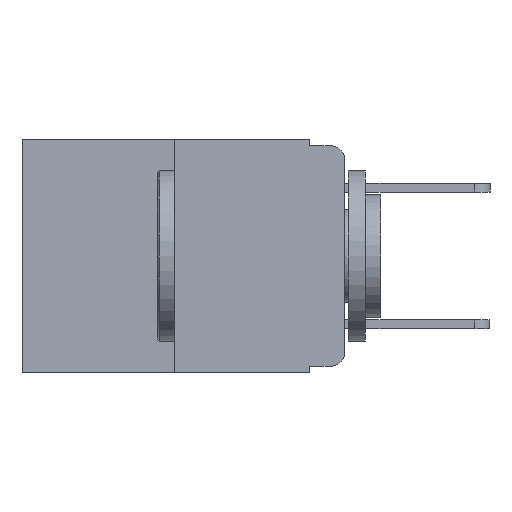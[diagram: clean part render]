
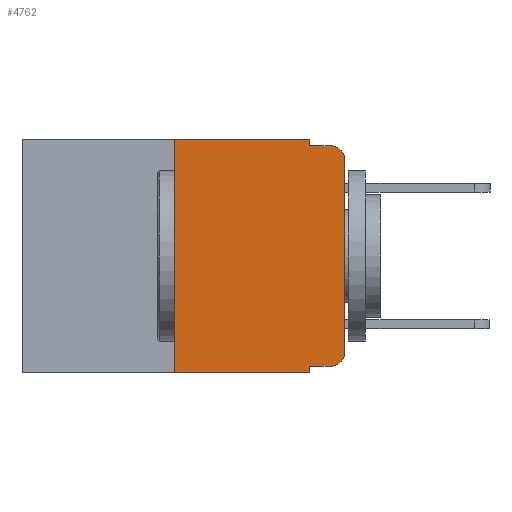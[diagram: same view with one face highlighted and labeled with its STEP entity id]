
A CAD part, left-side view. The second image highlights one B-rep face of the part: STEP entity #4762.
In plain terms, the highlighted planar face has unit normal (-1, 0, 0).
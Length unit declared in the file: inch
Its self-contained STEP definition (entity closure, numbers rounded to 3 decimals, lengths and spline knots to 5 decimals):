
#16 = ORIENTED_EDGE ( 'NONE', *, *, #5160, .F. ) ;
#153 = ORIENTED_EDGE ( 'NONE', *, *, #15971, .F. ) ;
#189 = AXIS2_PLACEMENT_3D ( 'NONE', #8895, #695, #12003 ) ;
#203 = ORIENTED_EDGE ( 'NONE', *, *, #5187, .F. ) ;
#223 = ORIENTED_EDGE ( 'NONE', *, *, #11264, .T. ) ;
#386 = VECTOR ( 'NONE', #772, 39.37008 ) ;
#425 = CIRCLE ( 'NONE', #189, 0.02 ) ;
#486 = ORIENTED_EDGE ( 'NONE', *, *, #5216, .F. ) ;
#529 = ORIENTED_EDGE ( 'NONE', *, *, #5248, .T. ) ;
#695 = DIRECTION ( 'NONE',  ( -1., 0., 0. ) ) ;
#772 = DIRECTION ( 'NONE',  ( 0., 0., 1. ) ) ;
#849 = CARTESIAN_POINT ( 'NONE',  ( 0., 0.051, -0.343 ) ) ;
#901 = ORIENTED_EDGE ( 'NONE', *, *, #5281, .T. ) ;
#1326 = VERTEX_POINT ( 'NONE', #10271 ) ;
#1379 = CARTESIAN_POINT ( 'NONE',  ( 0., 0.02, -0.333 ) ) ;
#1404 = CARTESIAN_POINT ( 'NONE',  ( 0., 0.051, -0.01 ) ) ;
#1521 = ORIENTED_EDGE ( 'NONE', *, *, #3767, .T. ) ;
#2048 = VECTOR ( 'NONE', #12965, 39.37008 ) ;
#2095 = DIRECTION ( 'NONE',  ( 1., 0., 0. ) ) ;
#2375 = EDGE_LOOP ( 'NONE', ( #1521, #2548, #7678, #16, #153, #203, #223, #486, #529, #901 ) ) ;
#2379 = VERTEX_POINT ( 'NONE', #1379 ) ;
#2535 = CARTESIAN_POINT ( 'NONE',  ( 0., 0.051, -0.01 ) ) ;
#2548 = ORIENTED_EDGE ( 'NONE', *, *, #4311, .T. ) ;
#2632 = VERTEX_POINT ( 'NONE', #16385 ) ;
#3217 = VECTOR ( 'NONE', #9694, 39.37008 ) ;
#3767 = EDGE_CURVE ( 'NONE', #12517, #16315, #13210, .T. ) ;
#3770 = AXIS2_PLACEMENT_3D ( 'NONE', #10000, #2095, #11197 ) ;
#3823 = FACE_OUTER_BOUND ( 'NONE', #2375, .T. ) ;
#4311 = EDGE_CURVE ( 'NONE', #16315, #15438, #425, .T. ) ;
#4473 = CARTESIAN_POINT ( 'NONE',  ( 0., 0.02, -0.01 ) ) ;
#4698 = VERTEX_POINT ( 'NONE', #849 ) ;
#4762 = ADVANCED_FACE ( 'NONE', ( #3823 ), #6247, .F. ) ;
#4824 = EDGE_CURVE ( 'NONE', #13267, #15438, #15745, .T. ) ;
#5026 = DIRECTION ( 'NONE',  ( 0., 0., -1. ) ) ;
#5160 = EDGE_CURVE ( 'NONE', #1326, #13267, #11373, .T. ) ;
#5187 = EDGE_CURVE ( 'NONE', #2632, #14732, #13727, .T. ) ;
#5216 = EDGE_CURVE ( 'NONE', #6037, #4698, #7793, .T. ) ;
#5248 = EDGE_CURVE ( 'NONE', #6037, #2379, #16460, .T. ) ;
#5281 = EDGE_CURVE ( 'NONE', #2379, #12517, #9546, .T. ) ;
#6037 = VERTEX_POINT ( 'NONE', #15031 ) ;
#6181 = DIRECTION ( 'NONE',  ( -1., 0., 0. ) ) ;
#6247 = PLANE ( 'NONE',  #3770 ) ;
#6738 = LINE ( 'NONE', #14217, #15903 ) ;
#6863 = CARTESIAN_POINT ( 'NONE',  ( 0., 0., -0.313 ) ) ;
#7253 = CARTESIAN_POINT ( 'NONE',  ( 0., 0.473, 0. ) ) ;
#7620 = CARTESIAN_POINT ( 'NONE',  ( 0., 0.051, -0.333 ) ) ;
#7678 = ORIENTED_EDGE ( 'NONE', *, *, #4824, .F. ) ;
#7793 = LINE ( 'NONE', #15938, #13350 ) ;
#8553 = DIRECTION ( 'NONE',  ( 0., -1., 0. ) ) ;
#8785 = CARTESIAN_POINT ( 'NONE',  ( 0., 0., 0. ) ) ;
#8895 = CARTESIAN_POINT ( 'NONE',  ( 0., 0.02, -0.03 ) ) ;
#9403 = CARTESIAN_POINT ( 'NONE',  ( 0., 0., -0.03 ) ) ;
#9546 = CIRCLE ( 'NONE', #9877, 0.02 ) ;
#9694 = DIRECTION ( 'NONE',  ( 0., 0., 1. ) ) ;
#9877 = AXIS2_PLACEMENT_3D ( 'NONE', #13436, #6181, #14580 ) ;
#10000 = CARTESIAN_POINT ( 'NONE',  ( 0., 0.473, 0. ) ) ;
#10223 = CARTESIAN_POINT ( 'NONE',  ( 0., 0.051, 0. ) ) ;
#10271 = CARTESIAN_POINT ( 'NONE',  ( 0., 0.051, 0. ) ) ;
#11197 = DIRECTION ( 'NONE',  ( 0., 0., -1. ) ) ;
#11264 = EDGE_CURVE ( 'NONE', #2632, #4698, #6738, .T. ) ;
#11373 = LINE ( 'NONE', #10223, #14431 ) ;
#12003 = DIRECTION ( 'NONE',  ( 0., 0., -1. ) ) ;
#12517 = VERTEX_POINT ( 'NONE', #6863 ) ;
#12602 = VECTOR ( 'NONE', #13546, 39.37008 ) ;
#12965 = DIRECTION ( 'NONE',  ( 0., -1., 0. ) ) ;
#13210 = LINE ( 'NONE', #8785, #3217 ) ;
#13267 = VERTEX_POINT ( 'NONE', #2535 ) ;
#13350 = VECTOR ( 'NONE', #5026, 39.37008 ) ;
#13436 = CARTESIAN_POINT ( 'NONE',  ( 0., 0.02, -0.313 ) ) ;
#13546 = DIRECTION ( 'NONE',  ( 0., -1., 0. ) ) ;
#13644 = VECTOR ( 'NONE', #8553, 39.37008 ) ;
#13647 = CARTESIAN_POINT ( 'NONE',  ( 0., 0.25, 0. ) ) ;
#13727 = LINE ( 'NONE', #13647, #386 ) ;
#13995 = LINE ( 'NONE', #7253, #13644 ) ;
#14044 = CARTESIAN_POINT ( 'NONE',  ( 0., 0.25, 0. ) ) ;
#14217 = CARTESIAN_POINT ( 'NONE',  ( 0., 0.473, -0.343 ) ) ;
#14431 = VECTOR ( 'NONE', #16036, 39.37008 ) ;
#14580 = DIRECTION ( 'NONE',  ( 0., 0., -1. ) ) ;
#14732 = VERTEX_POINT ( 'NONE', #14044 ) ;
#15031 = CARTESIAN_POINT ( 'NONE',  ( 0., 0.051, -0.333 ) ) ;
#15389 = DIRECTION ( 'NONE',  ( 0., -1., 0. ) ) ;
#15438 = VERTEX_POINT ( 'NONE', #4473 ) ;
#15745 = LINE ( 'NONE', #1404, #2048 ) ;
#15903 = VECTOR ( 'NONE', #15389, 39.37008 ) ;
#15938 = CARTESIAN_POINT ( 'NONE',  ( 0., 0.051, 0. ) ) ;
#15971 = EDGE_CURVE ( 'NONE', #14732, #1326, #13995, .T. ) ;
#16036 = DIRECTION ( 'NONE',  ( 0., 0., -1. ) ) ;
#16315 = VERTEX_POINT ( 'NONE', #9403 ) ;
#16385 = CARTESIAN_POINT ( 'NONE',  ( 0., 0.25, -0.343 ) ) ;
#16460 = LINE ( 'NONE', #7620, #12602 ) ;
